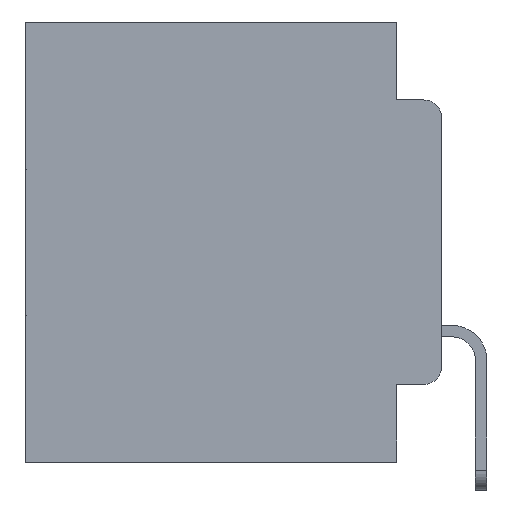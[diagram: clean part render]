
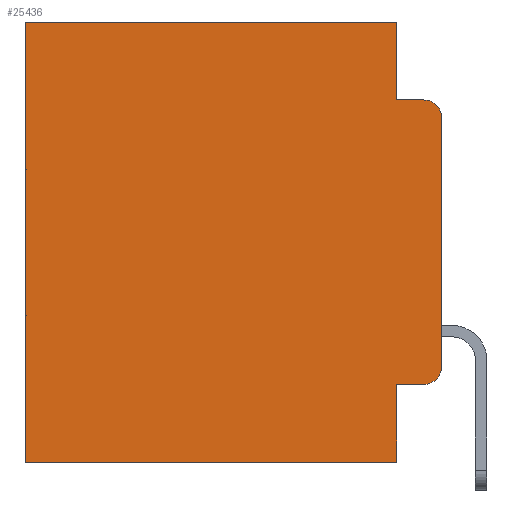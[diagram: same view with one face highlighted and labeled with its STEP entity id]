
A CAD part, left-side view. The second image highlights one B-rep face of the part: STEP entity #25436.
In plain terms, the highlighted planar face has unit normal (-1, 0, 0).
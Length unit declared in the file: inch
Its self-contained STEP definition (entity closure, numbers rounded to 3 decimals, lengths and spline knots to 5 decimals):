
#719 = CARTESIAN_POINT ( 'NONE',  ( 0.298, 0.473, 0. ) ) ;
#728 = AXIS2_PLACEMENT_3D ( 'NONE', #29709, #18786, #4901 ) ;
#915 = EDGE_CURVE ( 'NONE', #3034, #25296, #21772, .T. ) ;
#1049 = VECTOR ( 'NONE', #29692, 39.37008 ) ;
#1552 = CARTESIAN_POINT ( 'NONE',  ( 0.298, 0.051, 0. ) ) ;
#2113 = VERTEX_POINT ( 'NONE', #19970 ) ;
#2202 = CARTESIAN_POINT ( 'NONE',  ( 0.298, 0.02, -0.1085 ) ) ;
#2319 = VECTOR ( 'NONE', #29732, 39.37008 ) ;
#2417 = ORIENTED_EDGE ( 'NONE', *, *, #28403, .F. ) ;
#2652 = ORIENTED_EDGE ( 'NONE', *, *, #21948, .T. ) ;
#2786 = CARTESIAN_POINT ( 'NONE',  ( 0.298, 0.051, 0. ) ) ;
#2887 = ORIENTED_EDGE ( 'NONE', *, *, #7995, .F. ) ;
#3034 = VERTEX_POINT ( 'NONE', #4573 ) ;
#3268 = DIRECTION ( 'NONE',  ( 0., 0., -1. ) ) ;
#4573 = CARTESIAN_POINT ( 'NONE',  ( 0.298, 0.02, -0.4115 ) ) ;
#4767 = DIRECTION ( 'NONE',  ( 0., 0., -1. ) ) ;
#4901 = DIRECTION ( 'NONE',  ( 0., 0., -1. ) ) ;
#5012 = EDGE_CURVE ( 'NONE', #7195, #14481, #26206, .T. ) ;
#5667 = CARTESIAN_POINT ( 'NONE',  ( 0.298, 0.02, -0.0885 ) ) ;
#6258 = LINE ( 'NONE', #13358, #25151 ) ;
#7195 = VERTEX_POINT ( 'NONE', #14490 ) ;
#7510 = AXIS2_PLACEMENT_3D ( 'NONE', #2202, #18664, #4767 ) ;
#7995 = EDGE_CURVE ( 'NONE', #24006, #9234, #15869, .T. ) ;
#9193 = LINE ( 'NONE', #1552, #14646 ) ;
#9234 = VERTEX_POINT ( 'NONE', #13649 ) ;
#9740 = VECTOR ( 'NONE', #13651, 39.37008 ) ;
#9746 = CARTESIAN_POINT ( 'NONE',  ( 0.298, 0.051, -0.0885 ) ) ;
#10009 = LINE ( 'NONE', #719, #21335 ) ;
#10357 = VERTEX_POINT ( 'NONE', #2786 ) ;
#10624 = ORIENTED_EDGE ( 'NONE', *, *, #24727, .T. ) ;
#11310 = DIRECTION ( 'NONE',  ( 0., 0., -1. ) ) ;
#11344 = CARTESIAN_POINT ( 'NONE',  ( 0.298, 0., -0.3915 ) ) ;
#11551 = CARTESIAN_POINT ( 'NONE',  ( 0.298, 0.051, 0. ) ) ;
#11577 = CARTESIAN_POINT ( 'NONE',  ( 0.298, 0.051, -0.5 ) ) ;
#11681 = ORIENTED_EDGE ( 'NONE', *, *, #16501, .F. ) ;
#11892 = CIRCLE ( 'NONE', #7510, 0.02 ) ;
#12261 = DIRECTION ( 'NONE',  ( 0., 0., -1. ) ) ;
#12362 = VERTEX_POINT ( 'NONE', #14159 ) ;
#12950 = EDGE_CURVE ( 'NONE', #10357, #7195, #9193, .T. ) ;
#13356 = DIRECTION ( 'NONE',  ( 0., 1., 0. ) ) ;
#13358 = CARTESIAN_POINT ( 'NONE',  ( 0.298, 0., 0. ) ) ;
#13649 = CARTESIAN_POINT ( 'NONE',  ( 0.298, 0.473, -0.5 ) ) ;
#13651 = DIRECTION ( 'NONE',  ( 0., 1., 0. ) ) ;
#13810 = VECTOR ( 'NONE', #20635, 39.37008 ) ;
#14159 = CARTESIAN_POINT ( 'NONE',  ( 0.298, 0., -0.1085 ) ) ;
#14481 = VERTEX_POINT ( 'NONE', #5667 ) ;
#14490 = CARTESIAN_POINT ( 'NONE',  ( 0.298, 0.051, -0.0885 ) ) ;
#14584 = LINE ( 'NONE', #16546, #1049 ) ;
#14646 = VECTOR ( 'NONE', #11310, 39.37008 ) ;
#15095 = VERTEX_POINT ( 'NONE', #28358 ) ;
#15342 = ORIENTED_EDGE ( 'NONE', *, *, #5012, .F. ) ;
#15532 = EDGE_CURVE ( 'NONE', #15095, #3034, #14584, .T. ) ;
#15808 = ORIENTED_EDGE ( 'NONE', *, *, #24322, .T. ) ;
#15869 = LINE ( 'NONE', #29037, #9740 ) ;
#16348 = FACE_OUTER_BOUND ( 'NONE', #22046, .T. ) ;
#16461 = AXIS2_PLACEMENT_3D ( 'NONE', #17946, #22251, #12261 ) ;
#16501 = EDGE_CURVE ( 'NONE', #15095, #24006, #19793, .T. ) ;
#16546 = CARTESIAN_POINT ( 'NONE',  ( 0.298, 0.051, -0.4115 ) ) ;
#17810 = LINE ( 'NONE', #26762, #28209 ) ;
#17946 = CARTESIAN_POINT ( 'NONE',  ( 0.298, 0.02, -0.3915 ) ) ;
#18664 = DIRECTION ( 'NONE',  ( -1., 0., 0. ) ) ;
#18786 = DIRECTION ( 'NONE',  ( 1., 0., 0. ) ) ;
#19630 = ORIENTED_EDGE ( 'NONE', *, *, #915, .T. ) ;
#19793 = LINE ( 'NONE', #11551, #13810 ) ;
#19950 = ORIENTED_EDGE ( 'NONE', *, *, #15532, .T. ) ;
#19970 = CARTESIAN_POINT ( 'NONE',  ( 0.298, 0.473, 0. ) ) ;
#20600 = ORIENTED_EDGE ( 'NONE', *, *, #12950, .F. ) ;
#20635 = DIRECTION ( 'NONE',  ( 0., 0., -1. ) ) ;
#21335 = VECTOR ( 'NONE', #3268, 39.37008 ) ;
#21772 = CIRCLE ( 'NONE', #16461, 0.02 ) ;
#21948 = EDGE_CURVE ( 'NONE', #12362, #14481, #11892, .T. ) ;
#22046 = EDGE_LOOP ( 'NONE', ( #2417, #2652, #15342, #20600, #10624, #15808, #2887, #11681, #19950, #19630 ) ) ;
#22251 = DIRECTION ( 'NONE',  ( -1., 0., 0. ) ) ;
#24006 = VERTEX_POINT ( 'NONE', #11577 ) ;
#24322 = EDGE_CURVE ( 'NONE', #2113, #9234, #10009, .T. ) ;
#24727 = EDGE_CURVE ( 'NONE', #10357, #2113, #17810, .T. ) ;
#25151 = VECTOR ( 'NONE', #28841, 39.37008 ) ;
#25296 = VERTEX_POINT ( 'NONE', #11344 ) ;
#25436 = ADVANCED_FACE ( 'NONE', ( #16348 ), #27648, .F. ) ;
#26206 = LINE ( 'NONE', #9746, #2319 ) ;
#26762 = CARTESIAN_POINT ( 'NONE',  ( 0.298, 0., 0. ) ) ;
#27648 = PLANE ( 'NONE',  #728 ) ;
#28209 = VECTOR ( 'NONE', #13356, 39.37008 ) ;
#28358 = CARTESIAN_POINT ( 'NONE',  ( 0.298, 0.051, -0.4115 ) ) ;
#28403 = EDGE_CURVE ( 'NONE', #12362, #25296, #6258, .T. ) ;
#28841 = DIRECTION ( 'NONE',  ( 0., 0., -1. ) ) ;
#29037 = CARTESIAN_POINT ( 'NONE',  ( 0.298, 0., -0.5 ) ) ;
#29692 = DIRECTION ( 'NONE',  ( 0., -1., 0. ) ) ;
#29709 = CARTESIAN_POINT ( 'NONE',  ( 0.298, 0., 0. ) ) ;
#29732 = DIRECTION ( 'NONE',  ( 0., -1., 0. ) ) ;
